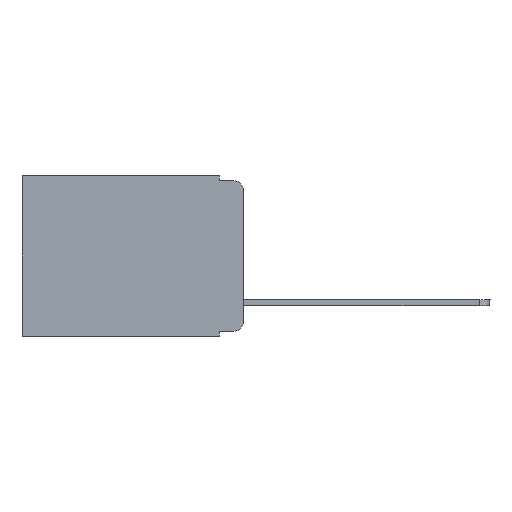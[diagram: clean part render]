
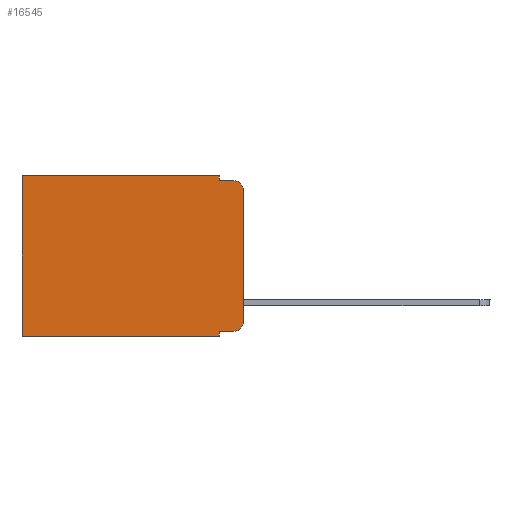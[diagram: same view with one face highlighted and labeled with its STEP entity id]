
A CAD part, left-side view. The second image highlights one B-rep face of the part: STEP entity #16545.
In plain terms, the highlighted planar face has unit normal (-1, 0, 0).
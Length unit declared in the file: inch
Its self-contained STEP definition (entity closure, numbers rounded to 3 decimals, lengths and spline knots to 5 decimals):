
#34 = VECTOR ( 'NONE', #10323, 39.37008 ) ;
#184 = EDGE_CURVE ( 'NONE', #7167, #387, #4718, .T. ) ;
#387 = VERTEX_POINT ( 'NONE', #14379 ) ;
#455 = CARTESIAN_POINT ( 'NONE',  ( 0.298, 0.051, 0. ) ) ;
#579 = CARTESIAN_POINT ( 'NONE',  ( 0.298, 0.051, -0.333 ) ) ;
#675 = DIRECTION ( 'NONE',  ( 0., 1., 0. ) ) ;
#727 = CARTESIAN_POINT ( 'NONE',  ( 0.298, 0.02, -0.333 ) ) ;
#835 = VECTOR ( 'NONE', #6203, 39.37008 ) ;
#854 = CIRCLE ( 'NONE', #3072, 0.02 ) ;
#1268 = CARTESIAN_POINT ( 'NONE',  ( 0.298, 0., 0. ) ) ;
#1362 = DIRECTION ( 'NONE',  ( 0., 0., -1. ) ) ;
#1430 = VECTOR ( 'NONE', #12102, 39.37008 ) ;
#1471 = EDGE_CURVE ( 'NONE', #4532, #17018, #2121, .T. ) ;
#1761 = DIRECTION ( 'NONE',  ( 0., 0., -1. ) ) ;
#2121 = LINE ( 'NONE', #14111, #34 ) ;
#2249 = LINE ( 'NONE', #3284, #14072 ) ;
#2288 = DIRECTION ( 'NONE',  ( 0., -1., 0. ) ) ;
#2745 = ORIENTED_EDGE ( 'NONE', *, *, #3094, .T. ) ;
#2933 = VERTEX_POINT ( 'NONE', #9050 ) ;
#2957 = CIRCLE ( 'NONE', #15561, 0.02 ) ;
#3072 = AXIS2_PLACEMENT_3D ( 'NONE', #9587, #6862, #12228 ) ;
#3094 = EDGE_CURVE ( 'NONE', #4532, #387, #2957, .T. ) ;
#3284 = CARTESIAN_POINT ( 'NONE',  ( 0.298, 0., -0.343 ) ) ;
#3567 = VERTEX_POINT ( 'NONE', #579 ) ;
#3797 = LINE ( 'NONE', #1268, #10492 ) ;
#3809 = CARTESIAN_POINT ( 'NONE',  ( 0.298, 0., -0.03 ) ) ;
#3987 = CARTESIAN_POINT ( 'NONE',  ( 0.298, 0.473, 0. ) ) ;
#4532 = VERTEX_POINT ( 'NONE', #3809 ) ;
#4718 = LINE ( 'NONE', #10070, #835 ) ;
#4860 = VECTOR ( 'NONE', #5350, 39.37008 ) ;
#5350 = DIRECTION ( 'NONE',  ( 0., 0., -1. ) ) ;
#5406 = EDGE_LOOP ( 'NONE', ( #8875, #2745, #6803, #8880, #15029, #13749, #17196, #6099, #16693, #7528 ) ) ;
#5627 = VECTOR ( 'NONE', #5771, 39.37008 ) ;
#5762 = EDGE_CURVE ( 'NONE', #10208, #16401, #2249, .T. ) ;
#5771 = DIRECTION ( 'NONE',  ( 0., 0., -1. ) ) ;
#6099 = ORIENTED_EDGE ( 'NONE', *, *, #6565, .F. ) ;
#6200 = EDGE_CURVE ( 'NONE', #2933, #12839, #3797, .T. ) ;
#6203 = DIRECTION ( 'NONE',  ( 0., -1., 0. ) ) ;
#6565 = EDGE_CURVE ( 'NONE', #3567, #10208, #9916, .T. ) ;
#6803 = ORIENTED_EDGE ( 'NONE', *, *, #184, .F. ) ;
#6862 = DIRECTION ( 'NONE',  ( -1., 0., 0. ) ) ;
#7167 = VERTEX_POINT ( 'NONE', #10837 ) ;
#7184 = EDGE_CURVE ( 'NONE', #11518, #17018, #854, .T. ) ;
#7528 = ORIENTED_EDGE ( 'NONE', *, *, #7184, .T. ) ;
#7995 = LINE ( 'NONE', #13238, #1430 ) ;
#8021 = PLANE ( 'NONE',  #14378 ) ;
#8875 = ORIENTED_EDGE ( 'NONE', *, *, #1471, .F. ) ;
#8880 = ORIENTED_EDGE ( 'NONE', *, *, #12272, .F. ) ;
#9050 = CARTESIAN_POINT ( 'NONE',  ( 0.298, 0.051, 0. ) ) ;
#9157 = CARTESIAN_POINT ( 'NONE',  ( 0.298, 0., 0. ) ) ;
#9587 = CARTESIAN_POINT ( 'NONE',  ( 0.298, 0.02, -0.313 ) ) ;
#9916 = LINE ( 'NONE', #455, #5627 ) ;
#10070 = CARTESIAN_POINT ( 'NONE',  ( 0.298, 0.051, -0.01 ) ) ;
#10208 = VERTEX_POINT ( 'NONE', #16847 ) ;
#10323 = DIRECTION ( 'NONE',  ( 0., 0., -1. ) ) ;
#10492 = VECTOR ( 'NONE', #17304, 39.37008 ) ;
#10556 = FACE_OUTER_BOUND ( 'NONE', #5406, .T. ) ;
#10837 = CARTESIAN_POINT ( 'NONE',  ( 0.298, 0.051, -0.01 ) ) ;
#11125 = DIRECTION ( 'NONE',  ( -1., 0., 0. ) ) ;
#11518 = VERTEX_POINT ( 'NONE', #727 ) ;
#12102 = DIRECTION ( 'NONE',  ( 0., 0., -1. ) ) ;
#12228 = DIRECTION ( 'NONE',  ( 0., 0., -1. ) ) ;
#12272 = EDGE_CURVE ( 'NONE', #2933, #7167, #7995, .T. ) ;
#12839 = VERTEX_POINT ( 'NONE', #3987 ) ;
#13238 = CARTESIAN_POINT ( 'NONE',  ( 0.298, 0.051, 0. ) ) ;
#13252 = CARTESIAN_POINT ( 'NONE',  ( 0.298, 0.473, 0. ) ) ;
#13749 = ORIENTED_EDGE ( 'NONE', *, *, #16925, .T. ) ;
#13751 = CARTESIAN_POINT ( 'NONE',  ( 0.298, 0.02, -0.03 ) ) ;
#14072 = VECTOR ( 'NONE', #675, 39.37008 ) ;
#14111 = CARTESIAN_POINT ( 'NONE',  ( 0.298, 0., 0. ) ) ;
#14113 = LINE ( 'NONE', #16934, #15460 ) ;
#14341 = CARTESIAN_POINT ( 'NONE',  ( 0.298, 0.473, -0.343 ) ) ;
#14378 = AXIS2_PLACEMENT_3D ( 'NONE', #9157, #14509, #1362 ) ;
#14379 = CARTESIAN_POINT ( 'NONE',  ( 0.298, 0.02, -0.01 ) ) ;
#14509 = DIRECTION ( 'NONE',  ( 1., 0., 0. ) ) ;
#15029 = ORIENTED_EDGE ( 'NONE', *, *, #6200, .T. ) ;
#15179 = EDGE_CURVE ( 'NONE', #3567, #11518, #14113, .T. ) ;
#15260 = CARTESIAN_POINT ( 'NONE',  ( 0.298, 0., -0.313 ) ) ;
#15460 = VECTOR ( 'NONE', #2288, 39.37008 ) ;
#15561 = AXIS2_PLACEMENT_3D ( 'NONE', #13751, #11125, #1761 ) ;
#16401 = VERTEX_POINT ( 'NONE', #14341 ) ;
#16545 = ADVANCED_FACE ( 'NONE', ( #10556 ), #8021, .F. ) ;
#16693 = ORIENTED_EDGE ( 'NONE', *, *, #15179, .T. ) ;
#16847 = CARTESIAN_POINT ( 'NONE',  ( 0.298, 0.051, -0.343 ) ) ;
#16925 = EDGE_CURVE ( 'NONE', #12839, #16401, #17301, .T. ) ;
#16934 = CARTESIAN_POINT ( 'NONE',  ( 0.298, 0.051, -0.333 ) ) ;
#17018 = VERTEX_POINT ( 'NONE', #15260 ) ;
#17196 = ORIENTED_EDGE ( 'NONE', *, *, #5762, .F. ) ;
#17301 = LINE ( 'NONE', #13252, #4860 ) ;
#17304 = DIRECTION ( 'NONE',  ( 0., 1., 0. ) ) ;
